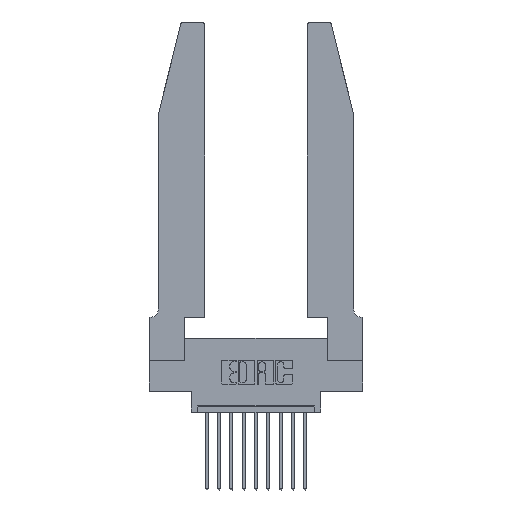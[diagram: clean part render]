
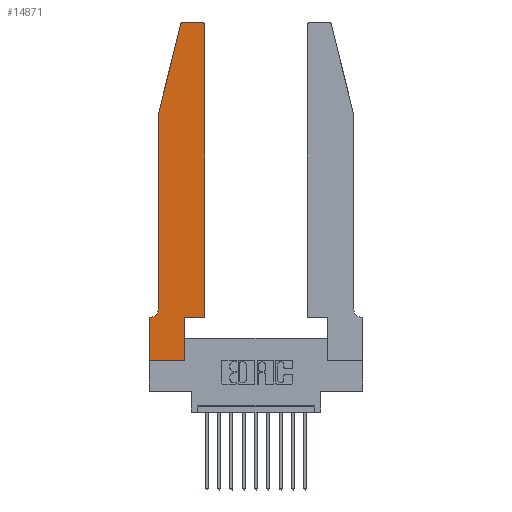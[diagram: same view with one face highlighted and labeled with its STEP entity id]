
A CAD part, top view. The second image highlights one B-rep face of the part: STEP entity #14871.
In plain terms, the highlighted planar face has unit normal (0, 0, 1).
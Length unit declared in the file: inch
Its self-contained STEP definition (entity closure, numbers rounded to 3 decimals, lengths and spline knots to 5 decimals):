
#252 = CARTESIAN_POINT ( 'NONE',  ( 0., 0., 0.37 ) ) ;
#385 = CARTESIAN_POINT ( 'NONE',  ( 0.2865, 0., 0.37 ) ) ;
#539 = VECTOR ( 'NONE', #3937, 39.37008 ) ;
#541 = ORIENTED_EDGE ( 'NONE', *, *, #11324, .T. ) ;
#560 = DIRECTION ( 'NONE',  ( -1., 0., 0. ) ) ;
#590 = FACE_OUTER_BOUND ( 'NONE', #3469, .T. ) ;
#655 = DIRECTION ( 'NONE',  ( 0., 0., 1. ) ) ;
#723 = CARTESIAN_POINT ( 'NONE',  ( 0., 0., 0.37 ) ) ;
#791 = CARTESIAN_POINT ( 'NONE',  ( 0.4205, 2.75, 0.37 ) ) ;
#827 = LINE ( 'NONE', #11572, #1989 ) ;
#988 = DIRECTION ( 'NONE',  ( 1., 0., 0. ) ) ;
#1344 = DIRECTION ( 'NONE',  ( 1., 0., 0. ) ) ;
#1468 = VERTEX_POINT ( 'NONE', #14048 ) ;
#1494 = VERTEX_POINT ( 'NONE', #723 ) ;
#1502 = AXIS2_PLACEMENT_3D ( 'NONE', #8759, #5156, #1344 ) ;
#1609 = AXIS2_PLACEMENT_3D ( 'NONE', #14260, #14312, #1870 ) ;
#1628 = CARTESIAN_POINT ( 'NONE',  ( 0.4505, 0.35, 0.37 ) ) ;
#1661 = AXIS2_PLACEMENT_3D ( 'NONE', #15229, #11666, #7737 ) ;
#1870 = DIRECTION ( 'NONE',  ( -1., 0., 0. ) ) ;
#1989 = VECTOR ( 'NONE', #4146, 39.37008 ) ;
#2092 = VERTEX_POINT ( 'NONE', #7056 ) ;
#2255 = CIRCLE ( 'NONE', #5412, 0.03 ) ;
#2275 = EDGE_CURVE ( 'NONE', #1468, #5328, #15554, .T. ) ;
#2412 = VERTEX_POINT ( 'NONE', #1628 ) ;
#2615 = DIRECTION ( 'NONE',  ( 0., -1., 0. ) ) ;
#2851 = ORIENTED_EDGE ( 'NONE', *, *, #15681, .T. ) ;
#2895 = LINE ( 'NONE', #252, #5797 ) ;
#2899 = EDGE_CURVE ( 'NONE', #4823, #1494, #2895, .T. ) ;
#2981 = LINE ( 'NONE', #13636, #4143 ) ;
#3469 = EDGE_LOOP ( 'NONE', ( #5694, #11777, #5409, #8928, #16078, #12341, #10082, #541, #8102, #16142, #2851, #3912 ) ) ;
#3475 = VECTOR ( 'NONE', #14829, 39.37008 ) ;
#3912 = ORIENTED_EDGE ( 'NONE', *, *, #10562, .T. ) ;
#3937 = DIRECTION ( 'NONE',  ( 0., 1., 0. ) ) ;
#4143 = VECTOR ( 'NONE', #5877, 39.37008 ) ;
#4146 = DIRECTION ( 'NONE',  ( -1., 0., 0. ) ) ;
#4184 = VECTOR ( 'NONE', #988, 39.37008 ) ;
#4369 = DIRECTION ( 'NONE',  ( 1., 0., 0. ) ) ;
#4413 = EDGE_CURVE ( 'NONE', #8166, #9750, #15727, .T. ) ;
#4823 = VERTEX_POINT ( 'NONE', #7807 ) ;
#4917 = CARTESIAN_POINT ( 'NONE',  ( 0.4505, 0.35, 0.37 ) ) ;
#4983 = VECTOR ( 'NONE', #9389, 39.37008 ) ;
#5156 = DIRECTION ( 'NONE',  ( 0., 0., 1. ) ) ;
#5229 = VERTEX_POINT ( 'NONE', #385 ) ;
#5312 = CARTESIAN_POINT ( 'NONE',  ( 0.284, 2.75, 0.37 ) ) ;
#5318 = EDGE_CURVE ( 'NONE', #9750, #1468, #2255, .T. ) ;
#5328 = VERTEX_POINT ( 'NONE', #5423 ) ;
#5409 = ORIENTED_EDGE ( 'NONE', *, *, #2275, .T. ) ;
#5412 = AXIS2_PLACEMENT_3D ( 'NONE', #9319, #655, #4369 ) ;
#5423 = CARTESIAN_POINT ( 'NONE',  ( 0.0755, 2., 0.37 ) ) ;
#5694 = ORIENTED_EDGE ( 'NONE', *, *, #4413, .T. ) ;
#5797 = VECTOR ( 'NONE', #2615, 39.37008 ) ;
#5877 = DIRECTION ( 'NONE',  ( 1., 0., 0. ) ) ;
#5886 = VERTEX_POINT ( 'NONE', #12800 ) ;
#6484 = LINE ( 'NONE', #10960, #4184 ) ;
#6766 = VERTEX_POINT ( 'NONE', #13906 ) ;
#6894 = EDGE_CURVE ( 'NONE', #2092, #2412, #2981, .T. ) ;
#7056 = CARTESIAN_POINT ( 'NONE',  ( 0.2865, 0.35, 0.37 ) ) ;
#7737 = DIRECTION ( 'NONE',  ( 1., 0., 0. ) ) ;
#7807 = CARTESIAN_POINT ( 'NONE',  ( 0., 0.35, 0.37 ) ) ;
#8102 = ORIENTED_EDGE ( 'NONE', *, *, #16114, .T. ) ;
#8136 = CARTESIAN_POINT ( 'NONE',  ( 0.0755, 2., 0.37 ) ) ;
#8166 = VERTEX_POINT ( 'NONE', #791 ) ;
#8759 = CARTESIAN_POINT ( 'NONE',  ( 0.4205, 2.72, 0.37 ) ) ;
#8928 = ORIENTED_EDGE ( 'NONE', *, *, #10398, .T. ) ;
#8947 = CARTESIAN_POINT ( 'NONE',  ( 0.0055, 0.35, 0.37 ) ) ;
#9219 = CIRCLE ( 'NONE', #1502, 0.03 ) ;
#9319 = CARTESIAN_POINT ( 'NONE',  ( 0.284, 2.72, 0.37 ) ) ;
#9389 = DIRECTION ( 'NONE',  ( 0., -1., 0. ) ) ;
#9406 = EDGE_CURVE ( 'NONE', #5886, #16075, #12420, .T. ) ;
#9750 = VERTEX_POINT ( 'NONE', #5312 ) ;
#10082 = ORIENTED_EDGE ( 'NONE', *, *, #2899, .T. ) ;
#10398 = EDGE_CURVE ( 'NONE', #5328, #5886, #15691, .T. ) ;
#10417 = PLANE ( 'NONE',  #1661 ) ;
#10562 = EDGE_CURVE ( 'NONE', #6766, #8166, #9219, .T. ) ;
#10960 = CARTESIAN_POINT ( 'NONE',  ( 0., 0., 0.37 ) ) ;
#11022 = CARTESIAN_POINT ( 'NONE',  ( 0.0755, 2., 0.37 ) ) ;
#11324 = EDGE_CURVE ( 'NONE', #1494, #5229, #6484, .T. ) ;
#11443 = VECTOR ( 'NONE', #13552, 39.37008 ) ;
#11572 = CARTESIAN_POINT ( 'NONE',  ( 0.0755, 0.35, 0.37 ) ) ;
#11636 = LINE ( 'NONE', #4917, #3475 ) ;
#11666 = DIRECTION ( 'NONE',  ( 0., 0., 1. ) ) ;
#11743 = CARTESIAN_POINT ( 'NONE',  ( 0.2605, 2.75, 0.37 ) ) ;
#11777 = ORIENTED_EDGE ( 'NONE', *, *, #5318, .T. ) ;
#11802 = LINE ( 'NONE', #13989, #539 ) ;
#12341 = ORIENTED_EDGE ( 'NONE', *, *, #12879, .T. ) ;
#12420 = CIRCLE ( 'NONE', #1609, 0.07 ) ;
#12800 = CARTESIAN_POINT ( 'NONE',  ( 0.0755, 0.42, 0.37 ) ) ;
#12879 = EDGE_CURVE ( 'NONE', #16075, #4823, #827, .T. ) ;
#13552 = DIRECTION ( 'NONE',  ( -0.239, -0.971, 0. ) ) ;
#13636 = CARTESIAN_POINT ( 'NONE',  ( 0.4505, 0.35, 0.37 ) ) ;
#13906 = CARTESIAN_POINT ( 'NONE',  ( 0.4505, 2.72, 0.37 ) ) ;
#13989 = CARTESIAN_POINT ( 'NONE',  ( 0.2865, 0.35, 0.37 ) ) ;
#14048 = CARTESIAN_POINT ( 'NONE',  ( 0.25487, 2.72718, 0.37 ) ) ;
#14154 = VECTOR ( 'NONE', #560, 39.37008 ) ;
#14260 = CARTESIAN_POINT ( 'NONE',  ( 0.0055, 0.42, 0.37 ) ) ;
#14312 = DIRECTION ( 'NONE',  ( 0., 0., -1. ) ) ;
#14829 = DIRECTION ( 'NONE',  ( 0., 1., 0. ) ) ;
#14871 = ADVANCED_FACE ( 'NONE', ( #590 ), #10417, .T. ) ;
#15229 = CARTESIAN_POINT ( 'NONE',  ( 0., 0.35, 0.37 ) ) ;
#15554 = LINE ( 'NONE', #11022, #11443 ) ;
#15681 = EDGE_CURVE ( 'NONE', #2412, #6766, #11636, .T. ) ;
#15691 = LINE ( 'NONE', #8136, #4983 ) ;
#15727 = LINE ( 'NONE', #11743, #14154 ) ;
#16075 = VERTEX_POINT ( 'NONE', #8947 ) ;
#16078 = ORIENTED_EDGE ( 'NONE', *, *, #9406, .T. ) ;
#16114 = EDGE_CURVE ( 'NONE', #5229, #2092, #11802, .T. ) ;
#16142 = ORIENTED_EDGE ( 'NONE', *, *, #6894, .T. ) ;
